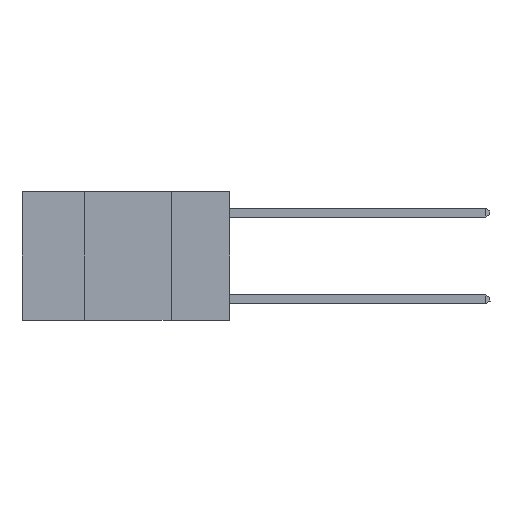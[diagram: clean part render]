
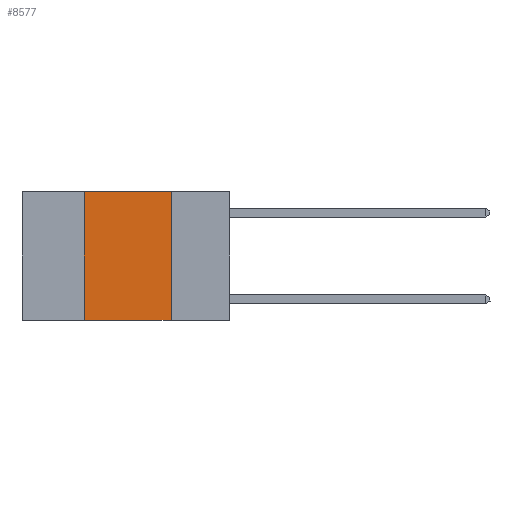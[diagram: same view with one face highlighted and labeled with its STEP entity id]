
A CAD part, left-side view. The second image highlights one B-rep face of the part: STEP entity #8577.
In plain terms, the highlighted planar face has unit normal (-1, 0, 0).
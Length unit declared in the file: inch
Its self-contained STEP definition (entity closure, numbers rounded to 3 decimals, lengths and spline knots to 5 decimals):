
#417 = VECTOR ( 'NONE', #2800, 39.37008 ) ;
#687 = PLANE ( 'NONE',  #5487 ) ;
#2800 = DIRECTION ( 'NONE',  ( 0., 0., -1. ) ) ;
#3996 = VERTEX_POINT ( 'NONE', #15657 ) ;
#4005 = VECTOR ( 'NONE', #13349, 39.37008 ) ;
#4304 = VECTOR ( 'NONE', #13703, 39.37008 ) ;
#4849 = DIRECTION ( 'NONE',  ( 1., 0., 0. ) ) ;
#5487 = AXIS2_PLACEMENT_3D ( 'NONE', #16949, #4849, #18849 ) ;
#5968 = LINE ( 'NONE', #20332, #10220 ) ;
#6472 = DIRECTION ( 'NONE',  ( 0., 0., 1. ) ) ;
#7174 = LINE ( 'NONE', #24516, #417 ) ;
#8577 = ADVANCED_FACE ( 'NONE', ( #25116 ), #687, .F. ) ;
#9651 = CARTESIAN_POINT ( 'NONE',  ( 0., 0.6, -0.37 ) ) ;
#9971 = VERTEX_POINT ( 'NONE', #18231 ) ;
#10220 = VECTOR ( 'NONE', #6472, 39.37008 ) ;
#11126 = ORIENTED_EDGE ( 'NONE', *, *, #18789, .T. ) ;
#11605 = VERTEX_POINT ( 'NONE', #24292 ) ;
#13349 = DIRECTION ( 'NONE',  ( 0., -1., 0. ) ) ;
#13556 = ORIENTED_EDGE ( 'NONE', *, *, #15332, .F. ) ;
#13703 = DIRECTION ( 'NONE',  ( 0., -1., 0. ) ) ;
#14894 = LINE ( 'NONE', #22871, #4005 ) ;
#15332 = EDGE_CURVE ( 'NONE', #9971, #21136, #5968, .T. ) ;
#15657 = CARTESIAN_POINT ( 'NONE',  ( 0., 0.17, -0.37 ) ) ;
#16586 = EDGE_LOOP ( 'NONE', ( #17158, #20769, #13556, #11126 ) ) ;
#16949 = CARTESIAN_POINT ( 'NONE',  ( 0., 0.6, 0. ) ) ;
#17158 = ORIENTED_EDGE ( 'NONE', *, *, #17531, .F. ) ;
#17531 = EDGE_CURVE ( 'NONE', #11605, #3996, #7174, .T. ) ;
#18231 = CARTESIAN_POINT ( 'NONE',  ( 0., 0.42, -0.37 ) ) ;
#18789 = EDGE_CURVE ( 'NONE', #9971, #3996, #20265, .T. ) ;
#18849 = DIRECTION ( 'NONE',  ( 0., 0., -1. ) ) ;
#20265 = LINE ( 'NONE', #9651, #4304 ) ;
#20332 = CARTESIAN_POINT ( 'NONE',  ( 0., 0.42, 0. ) ) ;
#20769 = ORIENTED_EDGE ( 'NONE', *, *, #24865, .F. ) ;
#21136 = VERTEX_POINT ( 'NONE', #24812 ) ;
#22871 = CARTESIAN_POINT ( 'NONE',  ( 0., 0.6, 0. ) ) ;
#24292 = CARTESIAN_POINT ( 'NONE',  ( 0., 0.17, 0. ) ) ;
#24516 = CARTESIAN_POINT ( 'NONE',  ( 0., 0.17, 0. ) ) ;
#24812 = CARTESIAN_POINT ( 'NONE',  ( 0., 0.42, 0. ) ) ;
#24865 = EDGE_CURVE ( 'NONE', #21136, #11605, #14894, .T. ) ;
#25116 = FACE_OUTER_BOUND ( 'NONE', #16586, .T. ) ;
